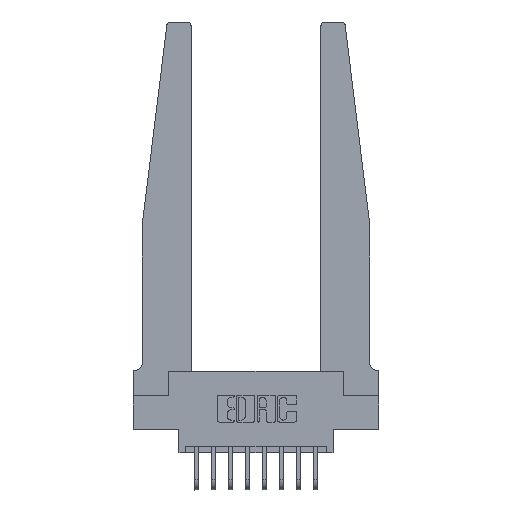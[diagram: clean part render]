
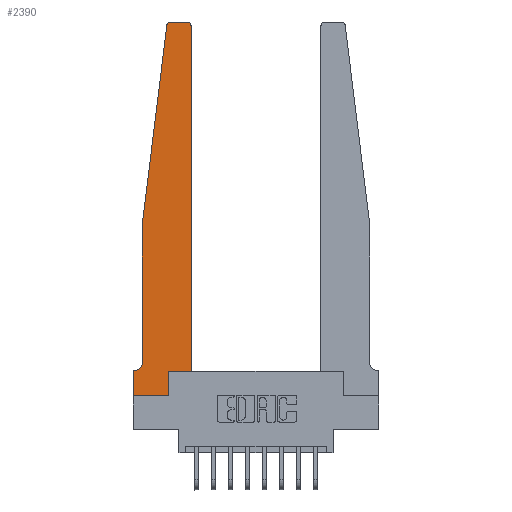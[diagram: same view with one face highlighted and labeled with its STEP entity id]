
A CAD part, top view. The second image highlights one B-rep face of the part: STEP entity #2390.
In plain terms, the highlighted planar face has unit normal (0, 0, 1).
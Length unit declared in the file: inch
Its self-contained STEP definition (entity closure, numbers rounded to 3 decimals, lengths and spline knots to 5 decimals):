
#59 = CARTESIAN_POINT ( 'NONE',  ( 0.015, 0.1875, 0.37 ) ) ;
#78 = EDGE_CURVE ( 'NONE', #1079, #11390, #11185, .T. ) ;
#360 = ORIENTED_EDGE ( 'NONE', *, *, #78, .T. ) ;
#502 = CARTESIAN_POINT ( 'NONE',  ( 0.395, 2.75, 0.37 ) ) ;
#549 = DIRECTION ( 'NONE',  ( 1., 0., 0. ) ) ;
#620 = VECTOR ( 'NONE', #1328, 39.37008 ) ;
#860 = EDGE_CURVE ( 'NONE', #8827, #1373, #2955, .T. ) ;
#901 = AXIS2_PLACEMENT_3D ( 'NONE', #9458, #2750, #10571 ) ;
#910 = DIRECTION ( 'NONE',  ( 0., 1., 0. ) ) ;
#1079 = VERTEX_POINT ( 'NONE', #3092 ) ;
#1328 = DIRECTION ( 'NONE',  ( 1., 0., 0. ) ) ;
#1373 = VERTEX_POINT ( 'NONE', #4826 ) ;
#1375 = VECTOR ( 'NONE', #13748, 39.37008 ) ;
#1851 = DIRECTION ( 'NONE',  ( -1., 0., 0. ) ) ;
#2277 = DIRECTION ( 'NONE',  ( -0.122, -0.992, 0. ) ) ;
#2390 = ADVANCED_FACE ( 'NONE', ( #11124 ), #8815, .T. ) ;
#2642 = LINE ( 'NONE', #14292, #8244 ) ;
#2678 = LINE ( 'NONE', #9159, #14168 ) ;
#2750 = DIRECTION ( 'NONE',  ( 0., 0., 1. ) ) ;
#2955 = CIRCLE ( 'NONE', #901, 0.03 ) ;
#3046 = CARTESIAN_POINT ( 'NONE',  ( 0.2605, 0.18, 0.37 ) ) ;
#3092 = CARTESIAN_POINT ( 'NONE',  ( 0.065, 0.2375, 0.37 ) ) ;
#3315 = AXIS2_PLACEMENT_3D ( 'NONE', #6596, #14373, #7737 ) ;
#3421 = ORIENTED_EDGE ( 'NONE', *, *, #3863, .T. ) ;
#3684 = LINE ( 'NONE', #8052, #620 ) ;
#3863 = EDGE_CURVE ( 'NONE', #3987, #1079, #5136, .T. ) ;
#3887 = VERTEX_POINT ( 'NONE', #12315 ) ;
#3987 = VERTEX_POINT ( 'NONE', #5813 ) ;
#4212 = CARTESIAN_POINT ( 'NONE',  ( 0.015, 0.2375, 0.37 ) ) ;
#4334 = CARTESIAN_POINT ( 'NONE',  ( 0.065, 0.1875, 0.37 ) ) ;
#4425 = EDGE_CURVE ( 'NONE', #7576, #5484, #2642, .T. ) ;
#4440 = CARTESIAN_POINT ( 'NONE',  ( 0.425, 0.18, 0.37 ) ) ;
#4441 = CARTESIAN_POINT ( 'NONE',  ( 0.065, 1.25, 0.37 ) ) ;
#4770 = CARTESIAN_POINT ( 'NONE',  ( 0., 0.1875, 0.37 ) ) ;
#4826 = CARTESIAN_POINT ( 'NONE',  ( 0.24675, 2.72367, 0.37 ) ) ;
#4884 = CARTESIAN_POINT ( 'NONE',  ( 0.25, 2.75, 0.37 ) ) ;
#5097 = CARTESIAN_POINT ( 'NONE',  ( 0.2605, 0., 0.37 ) ) ;
#5136 = LINE ( 'NONE', #4441, #10697 ) ;
#5325 = VERTEX_POINT ( 'NONE', #8323 ) ;
#5484 = VERTEX_POINT ( 'NONE', #3046 ) ;
#5494 = DIRECTION ( 'NONE',  ( 0., -1., 0. ) ) ;
#5813 = CARTESIAN_POINT ( 'NONE',  ( 0.065, 1.25, 0.37 ) ) ;
#6164 = EDGE_CURVE ( 'NONE', #11390, #11991, #8741, .T. ) ;
#6291 = AXIS2_PLACEMENT_3D ( 'NONE', #4212, #12544, #1851 ) ;
#6376 = ORIENTED_EDGE ( 'NONE', *, *, #9634, .T. ) ;
#6596 = CARTESIAN_POINT ( 'NONE',  ( 0., 0.1875, 0.37 ) ) ;
#6690 = CARTESIAN_POINT ( 'NONE',  ( 0.425, 2.72, 0.37 ) ) ;
#6701 = CARTESIAN_POINT ( 'NONE',  ( 0.065, 1.25, 0.37 ) ) ;
#7282 = DIRECTION ( 'NONE',  ( 0., -1., 0. ) ) ;
#7309 = DIRECTION ( 'NONE',  ( 0., 0., 1. ) ) ;
#7342 = LINE ( 'NONE', #4884, #1375 ) ;
#7424 = LINE ( 'NONE', #13942, #10386 ) ;
#7576 = VERTEX_POINT ( 'NONE', #5097 ) ;
#7663 = DIRECTION ( 'NONE',  ( -1., 0., 0. ) ) ;
#7737 = DIRECTION ( 'NONE',  ( 1., 0., 0. ) ) ;
#7793 = ORIENTED_EDGE ( 'NONE', *, *, #13886, .T. ) ;
#7846 = EDGE_CURVE ( 'NONE', #1373, #3987, #13565, .T. ) ;
#7962 = ORIENTED_EDGE ( 'NONE', *, *, #4425, .T. ) ;
#8052 = CARTESIAN_POINT ( 'NONE',  ( 0.425, 0.18, 0.37 ) ) ;
#8244 = VECTOR ( 'NONE', #910, 39.37008 ) ;
#8323 = CARTESIAN_POINT ( 'NONE',  ( 0., 0., 0.37 ) ) ;
#8741 = LINE ( 'NONE', #4334, #10999 ) ;
#8815 = PLANE ( 'NONE',  #3315 ) ;
#8827 = VERTEX_POINT ( 'NONE', #10877 ) ;
#8989 = ORIENTED_EDGE ( 'NONE', *, *, #13078, .T. ) ;
#9159 = CARTESIAN_POINT ( 'NONE',  ( 0., 0., 0.37 ) ) ;
#9378 = ORIENTED_EDGE ( 'NONE', *, *, #9903, .T. ) ;
#9458 = CARTESIAN_POINT ( 'NONE',  ( 0.27653, 2.72, 0.37 ) ) ;
#9504 = EDGE_LOOP ( 'NONE', ( #8989, #11004, #11963, #3421, #360, #9710, #6376, #14212, #7962, #9725, #9378, #7793 ) ) ;
#9523 = VECTOR ( 'NONE', #11073, 39.37008 ) ;
#9634 = EDGE_CURVE ( 'NONE', #11991, #5325, #7424, .T. ) ;
#9710 = ORIENTED_EDGE ( 'NONE', *, *, #6164, .T. ) ;
#9725 = ORIENTED_EDGE ( 'NONE', *, *, #13624, .T. ) ;
#9771 = CIRCLE ( 'NONE', #12484, 0.03 ) ;
#9903 = EDGE_CURVE ( 'NONE', #3887, #12979, #12133, .T. ) ;
#10386 = VECTOR ( 'NONE', #7282, 39.37008 ) ;
#10571 = DIRECTION ( 'NONE',  ( 1., 0., 0. ) ) ;
#10620 = VECTOR ( 'NONE', #2277, 39.37008 ) ;
#10697 = VECTOR ( 'NONE', #5494, 39.37008 ) ;
#10877 = CARTESIAN_POINT ( 'NONE',  ( 0.27653, 2.75, 0.37 ) ) ;
#10999 = VECTOR ( 'NONE', #7663, 39.37008 ) ;
#11004 = ORIENTED_EDGE ( 'NONE', *, *, #860, .T. ) ;
#11073 = DIRECTION ( 'NONE',  ( 0., 1., 0. ) ) ;
#11124 = FACE_OUTER_BOUND ( 'NONE', #9504, .T. ) ;
#11185 = CIRCLE ( 'NONE', #6291, 0.05 ) ;
#11310 = EDGE_CURVE ( 'NONE', #5325, #7576, #2678, .T. ) ;
#11390 = VERTEX_POINT ( 'NONE', #59 ) ;
#11963 = ORIENTED_EDGE ( 'NONE', *, *, #7846, .T. ) ;
#11991 = VERTEX_POINT ( 'NONE', #4770 ) ;
#12133 = LINE ( 'NONE', #4440, #9523 ) ;
#12315 = CARTESIAN_POINT ( 'NONE',  ( 0.425, 0.18, 0.37 ) ) ;
#12484 = AXIS2_PLACEMENT_3D ( 'NONE', #13967, #7309, #549 ) ;
#12544 = DIRECTION ( 'NONE',  ( 0., 0., -1. ) ) ;
#12979 = VERTEX_POINT ( 'NONE', #6690 ) ;
#13078 = EDGE_CURVE ( 'NONE', #13850, #8827, #7342, .T. ) ;
#13565 = LINE ( 'NONE', #6701, #10620 ) ;
#13615 = DIRECTION ( 'NONE',  ( 1., 0., 0. ) ) ;
#13624 = EDGE_CURVE ( 'NONE', #5484, #3887, #3684, .T. ) ;
#13748 = DIRECTION ( 'NONE',  ( -1., 0., 0. ) ) ;
#13850 = VERTEX_POINT ( 'NONE', #502 ) ;
#13886 = EDGE_CURVE ( 'NONE', #12979, #13850, #9771, .T. ) ;
#13942 = CARTESIAN_POINT ( 'NONE',  ( 0., 0., 0.37 ) ) ;
#13967 = CARTESIAN_POINT ( 'NONE',  ( 0.395, 2.72, 0.37 ) ) ;
#14168 = VECTOR ( 'NONE', #13615, 39.37008 ) ;
#14212 = ORIENTED_EDGE ( 'NONE', *, *, #11310, .T. ) ;
#14292 = CARTESIAN_POINT ( 'NONE',  ( 0.2605, 0.18, 0.37 ) ) ;
#14373 = DIRECTION ( 'NONE',  ( 0., 0., 1. ) ) ;
